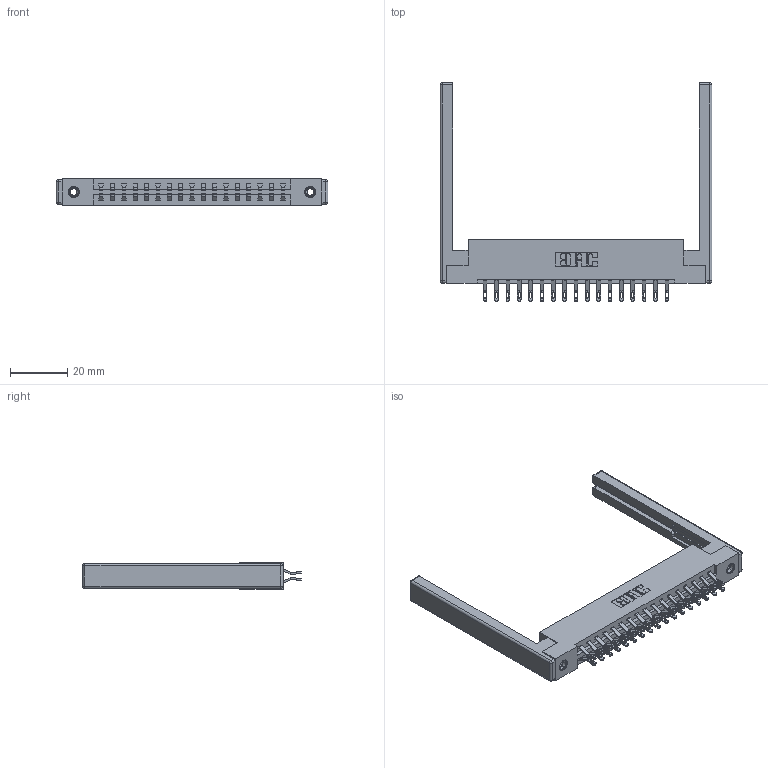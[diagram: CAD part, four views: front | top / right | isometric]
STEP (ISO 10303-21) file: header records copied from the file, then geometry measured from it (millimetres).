
FILE_DESCRIPTION (( 'STEP AP203' ), '1' );
FILE_NAME ('387-034-555-268.STEP', '2019-10-17T17:56:58', ( '' ), ( '' ), 'SwSTEP 2.0', 'SolidWorks 2016', '' );
FILE_SCHEMA (( 'CONFIG_CONTROL_DESIGN' ));
Length unit declared in the file: inch
Products named in the file (5): 337 Part_Flush Mounting Lugs - 0.156 Dia-TI; 387-034-555-268; 345-292-001_555 Tail; 307-220-068; 345-250-001_345-250-001-102
Assembly tree (39 placements, depth 2):
  387-034-555-268
    337 Part_Flush Mounting Lugs - 0.156 Dia-TI
    345-292-001_555 Tail  x34
    345-250-001_345-250-001-102  x2
    307-220-068  x2
Bounding box: 94.79 x 76.21 x 9.4 mm (x, y, z)
Volume: 14140.7 mm3; surface area: 15192.2 mm2
Topology: 39 solids, 39 shells, 2308 faces, 7127 edges, 4730 vertices
Faces by surface type: plane 1382, cylinder 902, cone 12, sphere 8, torus 4
Entity records: 19500 total; most frequent: CARTESIAN_POINT 3305, ORIENTED_EDGE 3200, DIRECTION 2898, EDGE_CURVE 1600, VECTOR 1402, LINE 1402, VERTEX_POINT 1058, AXIS2_PLACEMENT_3D 748
